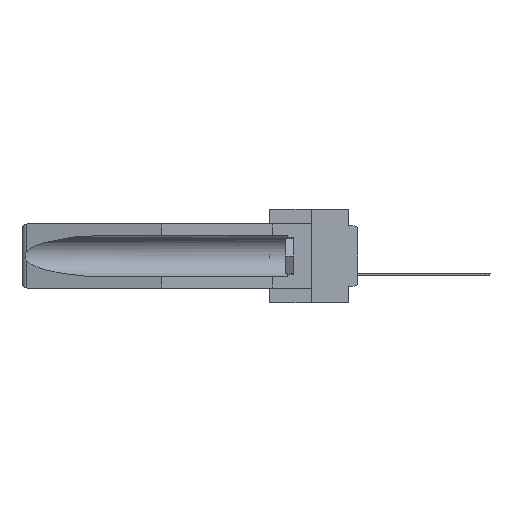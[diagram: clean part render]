
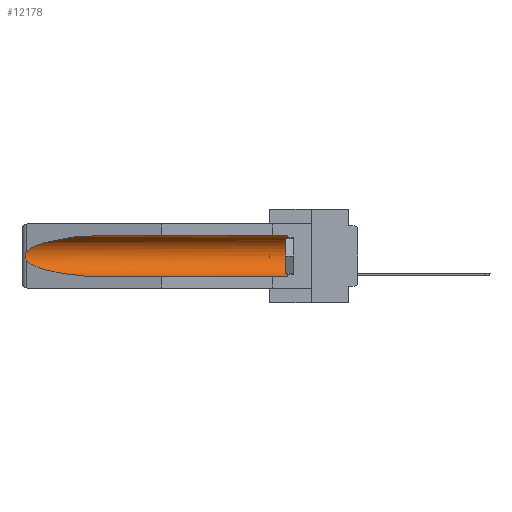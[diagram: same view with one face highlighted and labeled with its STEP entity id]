
A CAD part, left-side view. The second image highlights one B-rep face of the part: STEP entity #12178.
In plain terms, the highlighted cylindrical face has radius 2.857 mm (diameter 5.715 mm), a partial arc.
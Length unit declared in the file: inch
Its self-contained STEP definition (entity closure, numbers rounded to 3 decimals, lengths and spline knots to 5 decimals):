
#288 = VERTEX_POINT ( 'NONE', #22331 ) ;
#1037 = CARTESIAN_POINT ( 'NONE',  ( 0.26537, 1.52718, -0.14972 ) ) ;
#2025 = DIRECTION ( 'NONE',  ( 0., 1., 0. ) ) ;
#2671 = CARTESIAN_POINT ( 'NONE',  ( 0.26654, 1.53092, -0.15636 ) ) ;
#2905 = VECTOR ( 'NONE', #26361, 39.37008 ) ;
#2939 = ORIENTED_EDGE ( 'NONE', *, *, #35448, .T. ) ;
#3361 = LINE ( 'NONE', #35738, #2905 ) ;
#3805 = CARTESIAN_POINT ( 'NONE',  ( 0.21114, 1.30732, -0.059 ) ) ;
#3865 = AXIS2_PLACEMENT_3D ( 'NONE', #38624, #38489, #20523 ) ;
#4900 = CARTESIAN_POINT ( 'NONE',  ( 0.155, 0.126, -0.059 ) ) ;
#5729 = CARTESIAN_POINT ( 'NONE',  ( 0.2673, 1.5327, -0.16383 ) ) ;
#7104 = CARTESIAN_POINT ( 'NONE',  ( 0.25451, 1.48313, -0.09465 ) ) ;
#9318 = CARTESIAN_POINT ( 'NONE',  ( 0.26537, 1.52718, -0.19328 ) ) ;
#9530 = DIRECTION ( 'NONE',  ( 0., 1., 0. ) ) ;
#9667 = CARTESIAN_POINT ( 'NONE',  ( 0.155, 1.07973, -0.284 ) ) ;
#10878 = EDGE_LOOP ( 'NONE', ( #36608, #29731, #2939, #31142, #36557, #18099 ) ) ;
#11950 = EDGE_CURVE ( 'NONE', #34599, #12136, #30910, .T. ) ;
#12136 = VERTEX_POINT ( 'NONE', #24120 ) ;
#12178 = ADVANCED_FACE ( 'NONE', ( #17614 ), #25686, .F. ) ;
#12337 = CARTESIAN_POINT ( 'NONE',  ( 0.155, 1.07973, -0.059 ) ) ;
#12575 = CARTESIAN_POINT ( 'NONE',  ( 0.25451, 1.48313, -0.24835 ) ) ;
#14171 = CARTESIAN_POINT ( 'NONE',  ( 0.26597, 1.5296, -0.19026 ) ) ;
#14175 = CARTESIAN_POINT ( 'NONE',  ( 0.155, -0.30754, -0.284 ) ) ;
#14390 = B_SPLINE_CURVE_WITH_KNOTS ( 'NONE', 3,
 ( #26462, #29787, #2671, #5729, #14699, #26870, #29531, #32275, #14171, #20265 ),
 .UNSPECIFIED., .F., .F.,
 ( 4, 2, 2, 2, 4 ),
 ( 0., 0.00029, 0.00058, 0.00087, 0.00117 ),
 .UNSPECIFIED. ) ;
#14699 = CARTESIAN_POINT ( 'NONE',  ( 0.2675, 1.53308, -0.16763 ) ) ;
#17614 = FACE_OUTER_BOUND ( 'NONE', #10878, .T. ) ;
#18099 = ORIENTED_EDGE ( 'NONE', *, *, #28737, .T. ) ;
#19928 = AXIS2_PLACEMENT_3D ( 'NONE', #33451, #9530, #30691 ) ;
#20265 = CARTESIAN_POINT ( 'NONE',  ( 0.26537, 1.52718, -0.19328 ) ) ;
#20523 = DIRECTION ( 'NONE',  ( 0., 0., 1. ) ) ;
#21386 = CIRCLE ( 'NONE', #3865, 0.1125 ) ;
#22331 = CARTESIAN_POINT ( 'NONE',  ( 0.26537, 1.52718, -0.14972 ) ) ;
#24120 = CARTESIAN_POINT ( 'NONE',  ( 0.155, 1.07973, -0.284 ) ) ;
#24901 = CARTESIAN_POINT ( 'NONE',  ( 0.21114, 1.30732, -0.284 ) ) ;
#24991 = CARTESIAN_POINT ( 'NONE',  ( 0.155, 1.07973, -0.059 ) ) ;
#25686 = CYLINDRICAL_SURFACE ( 'NONE', #19928, 0.1125 ) ;
#25728 = VECTOR ( 'NONE', #2025, 39.37008 ) ;
#26111 = CARTESIAN_POINT ( 'NONE',  ( 0.155, 0.126, -0.284 ) ) ;
#26361 = DIRECTION ( 'NONE',  ( 0., 1., 0. ) ) ;
#26462 = CARTESIAN_POINT ( 'NONE',  ( 0.26537, 1.52718, -0.14972 ) ) ;
#26760 =( BOUNDED_CURVE ( )  B_SPLINE_CURVE ( 3, ( #30951, #12575, #24901, #9667 ),
 .UNSPECIFIED., .F., .F. ) 
 B_SPLINE_CURVE_WITH_KNOTS ( ( 4, 4 ),
 ( 0.1948, 1.5708 ),
 .UNSPECIFIED. ) 
 CURVE ( )  GEOMETRIC_REPRESENTATION_ITEM ( )  RATIONAL_B_SPLINE_CURVE ( ( 1., 0.848, 0.848, 1. ) ) 
 REPRESENTATION_ITEM ( '' )  );
#26870 = CARTESIAN_POINT ( 'NONE',  ( 0.2675, 1.53308, -0.17534 ) ) ;
#28305 = EDGE_CURVE ( 'NONE', #288, #36669, #14390, .T. ) ;
#28312 = EDGE_CURVE ( 'NONE', #34599, #38676, #21386, .T. ) ;
#28737 = EDGE_CURVE ( 'NONE', #38676, #34987, #3361, .T. ) ;
#29531 = CARTESIAN_POINT ( 'NONE',  ( 0.2673, 1.53269, -0.17917 ) ) ;
#29731 = ORIENTED_EDGE ( 'NONE', *, *, #28305, .T. ) ;
#29787 = CARTESIAN_POINT ( 'NONE',  ( 0.26597, 1.52961, -0.15275 ) ) ;
#30691 = DIRECTION ( 'NONE',  ( 0., 0., 1. ) ) ;
#30910 = LINE ( 'NONE', #14175, #25728 ) ;
#30951 = CARTESIAN_POINT ( 'NONE',  ( 0.26537, 1.52718, -0.19328 ) ) ;
#31142 = ORIENTED_EDGE ( 'NONE', *, *, #11950, .F. ) ;
#32275 = CARTESIAN_POINT ( 'NONE',  ( 0.26655, 1.53094, -0.18657 ) ) ;
#33451 = CARTESIAN_POINT ( 'NONE',  ( 0.155, -0.30754, -0.1715 ) ) ;
#34599 = VERTEX_POINT ( 'NONE', #26111 ) ;
#34987 = VERTEX_POINT ( 'NONE', #12337 ) ;
#35448 = EDGE_CURVE ( 'NONE', #36669, #12136, #26760, .T. ) ;
#35738 = CARTESIAN_POINT ( 'NONE',  ( 0.155, -0.30754, -0.059 ) ) ;
#36085 = EDGE_CURVE ( 'NONE', #34987, #288, #38384, .T. ) ;
#36557 = ORIENTED_EDGE ( 'NONE', *, *, #28312, .T. ) ;
#36608 = ORIENTED_EDGE ( 'NONE', *, *, #36085, .T. ) ;
#36669 = VERTEX_POINT ( 'NONE', #9318 ) ;
#38384 =( BOUNDED_CURVE ( )  B_SPLINE_CURVE ( 3, ( #24991, #3805, #7104, #1037 ),
 .UNSPECIFIED., .F., .F. ) 
 B_SPLINE_CURVE_WITH_KNOTS ( ( 4, 4 ),
 ( 4.71239, 6.08839 ),
 .UNSPECIFIED. ) 
 CURVE ( )  GEOMETRIC_REPRESENTATION_ITEM ( )  RATIONAL_B_SPLINE_CURVE ( ( 1., 0.848, 0.848, 1. ) ) 
 REPRESENTATION_ITEM ( '' )  );
#38489 = DIRECTION ( 'NONE',  ( 0., -1., 0. ) ) ;
#38624 = CARTESIAN_POINT ( 'NONE',  ( 0.155, 0.126, -0.1715 ) ) ;
#38676 = VERTEX_POINT ( 'NONE', #4900 ) ;
